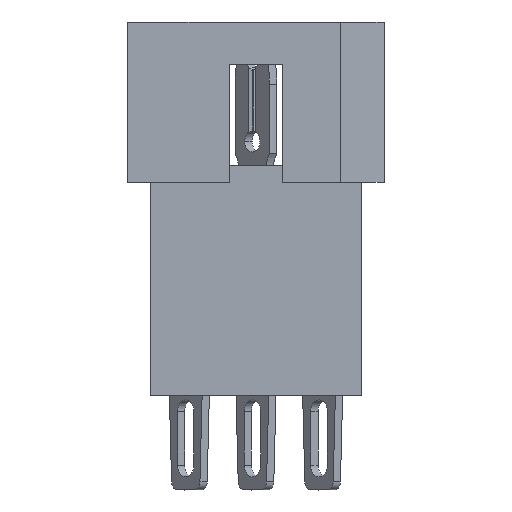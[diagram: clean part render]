
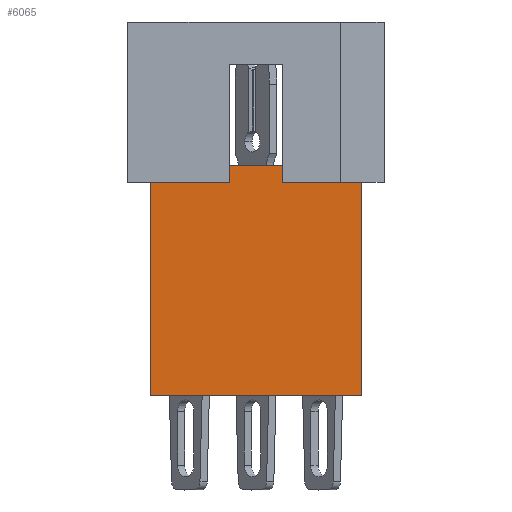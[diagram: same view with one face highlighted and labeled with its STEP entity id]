
A CAD part, top view. The second image highlights one B-rep face of the part: STEP entity #6065.
In plain terms, the highlighted planar face has unit normal (0, 0, 1).
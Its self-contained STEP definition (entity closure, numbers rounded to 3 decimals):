
#103 = LINE ( 'NONE', #5359, #5075 ) ;
#164 = DIRECTION ( 'NONE',  ( 0., 0., 1. ) ) ;
#239 = LINE ( 'NONE', #2936, #2120 ) ;
#262 = ORIENTED_EDGE ( 'NONE', *, *, #4735, .F. ) ;
#344 = CARTESIAN_POINT ( 'NONE',  ( 10.249, -12.7, 2.54 ) ) ;
#484 = ORIENTED_EDGE ( 'NONE', *, *, #1483, .F. ) ;
#599 = CARTESIAN_POINT ( 'NONE',  ( 2.362, 6.985, 2.54 ) ) ;
#745 = CARTESIAN_POINT ( 'NONE',  ( -2.324, 0., 2.54 ) ) ;
#866 = LINE ( 'NONE', #745, #4780 ) ;
#1079 = VERTEX_POINT ( 'NONE', #3784 ) ;
#1211 = VECTOR ( 'NONE', #5101, 1000. ) ;
#1274 = DIRECTION ( 'NONE',  ( 1., 0., 0. ) ) ;
#1483 = EDGE_CURVE ( 'NONE', #3080, #4240, #4079, .T. ) ;
#1484 = DIRECTION ( 'NONE',  ( 0., 1., 0. ) ) ;
#1821 = EDGE_CURVE ( 'NONE', #4446, #5874, #866, .T. ) ;
#1827 = ORIENTED_EDGE ( 'NONE', *, *, #3014, .T. ) ;
#1835 = ORIENTED_EDGE ( 'NONE', *, *, #2370, .T. ) ;
#1849 = VECTOR ( 'NONE', #1895, 1000. ) ;
#1895 = DIRECTION ( 'NONE',  ( 0., 1., 0. ) ) ;
#2006 = CARTESIAN_POINT ( 'NONE',  ( 5.563, 6.985, 2.54 ) ) ;
#2120 = VECTOR ( 'NONE', #4995, 1000. ) ;
#2263 = LINE ( 'NONE', #599, #4011 ) ;
#2370 = EDGE_CURVE ( 'NONE', #4809, #4240, #103, .T. ) ;
#2756 = CARTESIAN_POINT ( 'NONE',  ( -2.324, -12.7, 2.54 ) ) ;
#2840 = EDGE_CURVE ( 'NONE', #6148, #5874, #2263, .T. ) ;
#2877 = CARTESIAN_POINT ( 'NONE',  ( 2.362, 1.016, 2.54 ) ) ;
#2910 = AXIS2_PLACEMENT_3D ( 'NONE', #2756, #164, #1274 ) ;
#2926 = CARTESIAN_POINT ( 'NONE',  ( -2.324, -12.7, 2.54 ) ) ;
#2936 = CARTESIAN_POINT ( 'NONE',  ( -2.324, -12.7, 2.54 ) ) ;
#2984 = ORIENTED_EDGE ( 'NONE', *, *, #1821, .F. ) ;
#3014 = EDGE_CURVE ( 'NONE', #1079, #4809, #239, .T. ) ;
#3080 = VERTEX_POINT ( 'NONE', #5942 ) ;
#3095 = EDGE_CURVE ( 'NONE', #6148, #3372, #3621, .T. ) ;
#3159 = CARTESIAN_POINT ( 'NONE',  ( -2.324, 0., 2.54 ) ) ;
#3242 = PLANE ( 'NONE',  #2910 ) ;
#3372 = VERTEX_POINT ( 'NONE', #5817 ) ;
#3482 = DIRECTION ( 'NONE',  ( 1., 0., 0. ) ) ;
#3621 = LINE ( 'NONE', #6593, #4089 ) ;
#3784 = CARTESIAN_POINT ( 'NONE',  ( -2.324, -12.7, 2.54 ) ) ;
#3822 = LINE ( 'NONE', #2006, #4624 ) ;
#4011 = VECTOR ( 'NONE', #5250, 1000. ) ;
#4079 = LINE ( 'NONE', #6111, #1211 ) ;
#4089 = VECTOR ( 'NONE', #3482, 1000. ) ;
#4240 = VERTEX_POINT ( 'NONE', #6462 ) ;
#4271 = EDGE_LOOP ( 'NONE', ( #2984, #262, #1827, #1835, #484, #5390, #6351, #6276 ) ) ;
#4317 = DIRECTION ( 'NONE',  ( 1., 0., 0. ) ) ;
#4446 = VERTEX_POINT ( 'NONE', #3159 ) ;
#4464 = LINE ( 'NONE', #2926, #1849 ) ;
#4624 = VECTOR ( 'NONE', #1484, 1000. ) ;
#4735 = EDGE_CURVE ( 'NONE', #1079, #4446, #4464, .T. ) ;
#4780 = VECTOR ( 'NONE', #4317, 1000. ) ;
#4809 = VERTEX_POINT ( 'NONE', #344 ) ;
#4834 = DIRECTION ( 'NONE',  ( 0., 1., 0. ) ) ;
#4932 = FACE_OUTER_BOUND ( 'NONE', #4271, .T. ) ;
#4995 = DIRECTION ( 'NONE',  ( 1., 0., 0. ) ) ;
#5075 = VECTOR ( 'NONE', #4834, 1000. ) ;
#5101 = DIRECTION ( 'NONE',  ( 1., 0., 0. ) ) ;
#5162 = CARTESIAN_POINT ( 'NONE',  ( 2.362, 0., 2.54 ) ) ;
#5250 = DIRECTION ( 'NONE',  ( 0., -1., 0. ) ) ;
#5359 = CARTESIAN_POINT ( 'NONE',  ( 10.249, -12.7, 2.54 ) ) ;
#5390 = ORIENTED_EDGE ( 'NONE', *, *, #5398, .T. ) ;
#5398 = EDGE_CURVE ( 'NONE', #3080, #3372, #3822, .T. ) ;
#5817 = CARTESIAN_POINT ( 'NONE',  ( 5.563, 1.016, 2.54 ) ) ;
#5874 = VERTEX_POINT ( 'NONE', #5162 ) ;
#5942 = CARTESIAN_POINT ( 'NONE',  ( 5.563, 0., 2.54 ) ) ;
#6065 = ADVANCED_FACE ( 'NONE', ( #4932 ), #3242, .T. ) ;
#6111 = CARTESIAN_POINT ( 'NONE',  ( -2.324, 0., 2.54 ) ) ;
#6148 = VERTEX_POINT ( 'NONE', #2877 ) ;
#6276 = ORIENTED_EDGE ( 'NONE', *, *, #2840, .T. ) ;
#6351 = ORIENTED_EDGE ( 'NONE', *, *, #3095, .F. ) ;
#6462 = CARTESIAN_POINT ( 'NONE',  ( 10.249, 0., 2.54 ) ) ;
#6593 = CARTESIAN_POINT ( 'NONE',  ( 0., 1.016, 2.54 ) ) ;
